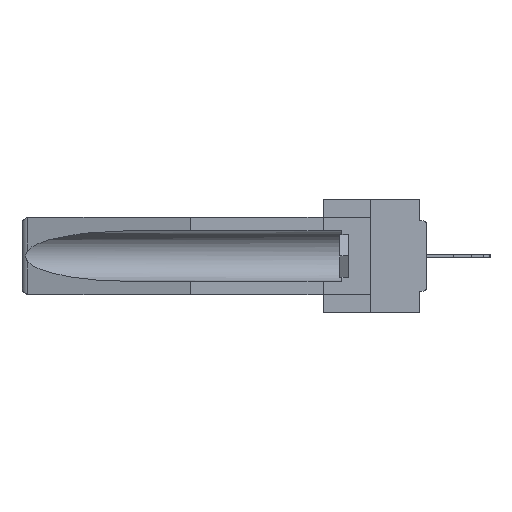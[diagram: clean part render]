
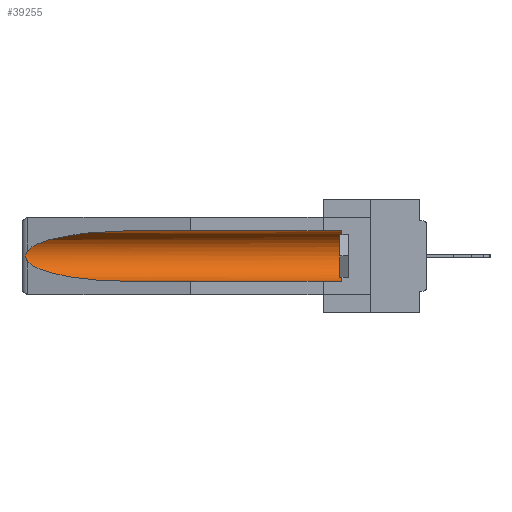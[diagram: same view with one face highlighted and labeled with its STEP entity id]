
A CAD part, left-side view. The second image highlights one B-rep face of the part: STEP entity #39255.
In plain terms, the highlighted cylindrical face has radius 2.857 mm (diameter 5.715 mm), a partial arc.
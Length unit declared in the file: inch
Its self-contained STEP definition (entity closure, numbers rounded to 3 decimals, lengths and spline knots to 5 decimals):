
#907 = CARTESIAN_POINT ( 'NONE',  ( 0.21114, 1.30732, -0.284 ) ) ;
#1145 = ORIENTED_EDGE ( 'NONE', *, *, #2730, .T. ) ;
#1500 = CARTESIAN_POINT ( 'NONE',  ( 0.155, 1.07973, -0.284 ) ) ;
#2730 = EDGE_CURVE ( 'NONE', #5577, #13444, #19659, .T. ) ;
#3007 = CARTESIAN_POINT ( 'NONE',  ( 0.26597, 1.5296, -0.19026 ) ) ;
#4577 = VERTEX_POINT ( 'NONE', #11105 ) ;
#5098 = VECTOR ( 'NONE', #37094, 39.37008 ) ;
#5509 = EDGE_CURVE ( 'NONE', #5577, #16531, #6895, .T. ) ;
#5577 = VERTEX_POINT ( 'NONE', #8643 ) ;
#5765 = CARTESIAN_POINT ( 'NONE',  ( 0.25451, 1.48313, -0.09465 ) ) ;
#6176 = CARTESIAN_POINT ( 'NONE',  ( 0.155, 1.07973, -0.059 ) ) ;
#6895 = LINE ( 'NONE', #29945, #38728 ) ;
#7158 = DIRECTION ( 'NONE',  ( 0., 1., 0. ) ) ;
#7533 = VERTEX_POINT ( 'NONE', #6176 ) ;
#7976 = ORIENTED_EDGE ( 'NONE', *, *, #5509, .F. ) ;
#8643 = CARTESIAN_POINT ( 'NONE',  ( 0.155, 0.126, -0.284 ) ) ;
#9172 = CARTESIAN_POINT ( 'NONE',  ( 0.26597, 1.52961, -0.15275 ) ) ;
#10484 = VERTEX_POINT ( 'NONE', #34458 ) ;
#11095 = DIRECTION ( 'NONE',  ( 0., -1., 0. ) ) ;
#11105 = CARTESIAN_POINT ( 'NONE',  ( 0.26537, 1.52718, -0.19328 ) ) ;
#11738 = B_SPLINE_CURVE_WITH_KNOTS ( 'NONE', 3,
 ( #18385, #9172, #33818, #15425, #36960, #18511, #40015, #21604, #3007, #24680 ),
 .UNSPECIFIED., .F., .F.,
 ( 4, 2, 2, 2, 4 ),
 ( 0., 0.00029, 0.00058, 0.00087, 0.00117 ),
 .UNSPECIFIED. ) ;
#13401 = LINE ( 'NONE', #21730, #5098 ) ;
#13444 = VERTEX_POINT ( 'NONE', #15749 ) ;
#13967 =( BOUNDED_CURVE ( )  B_SPLINE_CURVE ( 3, ( #38015, #19577, #907, #22663 ),
 .UNSPECIFIED., .F., .T. ) 
 B_SPLINE_CURVE_WITH_KNOTS ( ( 4, 4 ),
 ( 0.1948, 1.5708 ),
 .UNSPECIFIED. ) 
 CURVE ( )  GEOMETRIC_REPRESENTATION_ITEM ( )  RATIONAL_B_SPLINE_CURVE ( ( 1., 0.848, 0.848, 1. ) ) 
 REPRESENTATION_ITEM ( '' )  );
#14114 = AXIS2_PLACEMENT_3D ( 'NONE', #34916, #7158, #16513 ) ;
#14897 = ORIENTED_EDGE ( 'NONE', *, *, #30225, .T. ) ;
#15425 = CARTESIAN_POINT ( 'NONE',  ( 0.2673, 1.5327, -0.16383 ) ) ;
#15749 = CARTESIAN_POINT ( 'NONE',  ( 0.155, 0.126, -0.059 ) ) ;
#16513 = DIRECTION ( 'NONE',  ( 0., 0., 1. ) ) ;
#16531 = VERTEX_POINT ( 'NONE', #1500 ) ;
#16762 = EDGE_CURVE ( 'NONE', #7533, #10484, #32102, .T. ) ;
#16821 = EDGE_LOOP ( 'NONE', ( #34192, #40185, #24329, #7976, #1145, #14897 ) ) ;
#18385 = CARTESIAN_POINT ( 'NONE',  ( 0.26537, 1.52718, -0.14972 ) ) ;
#18511 = CARTESIAN_POINT ( 'NONE',  ( 0.2675, 1.53308, -0.17534 ) ) ;
#19577 = CARTESIAN_POINT ( 'NONE',  ( 0.25451, 1.48313, -0.24835 ) ) ;
#19659 = CIRCLE ( 'NONE', #37400, 0.1125 ) ;
#20816 = DIRECTION ( 'NONE',  ( 0., 1., 0. ) ) ;
#21604 = CARTESIAN_POINT ( 'NONE',  ( 0.26655, 1.53094, -0.18657 ) ) ;
#21730 = CARTESIAN_POINT ( 'NONE',  ( 0.155, -0.30754, -0.059 ) ) ;
#22663 = CARTESIAN_POINT ( 'NONE',  ( 0.155, 1.07973, -0.284 ) ) ;
#23661 = CYLINDRICAL_SURFACE ( 'NONE', #14114, 0.1125 ) ;
#24329 = ORIENTED_EDGE ( 'NONE', *, *, #34703, .T. ) ;
#24680 = CARTESIAN_POINT ( 'NONE',  ( 0.26537, 1.52718, -0.19328 ) ) ;
#27367 = CARTESIAN_POINT ( 'NONE',  ( 0.26537, 1.52718, -0.14972 ) ) ;
#28346 = EDGE_CURVE ( 'NONE', #10484, #4577, #11738, .T. ) ;
#29517 = CARTESIAN_POINT ( 'NONE',  ( 0.155, 0.126, -0.1715 ) ) ;
#29945 = CARTESIAN_POINT ( 'NONE',  ( 0.155, -0.30754, -0.284 ) ) ;
#30225 = EDGE_CURVE ( 'NONE', #13444, #7533, #13401, .T. ) ;
#30353 = CARTESIAN_POINT ( 'NONE',  ( 0.155, 1.07973, -0.059 ) ) ;
#32102 =( BOUNDED_CURVE ( )  B_SPLINE_CURVE ( 3, ( #30353, #33426, #5765, #27367 ),
 .UNSPECIFIED., .F., .F. ) 
 B_SPLINE_CURVE_WITH_KNOTS ( ( 4, 4 ),
 ( 4.71239, 6.08839 ),
 .UNSPECIFIED. ) 
 CURVE ( )  GEOMETRIC_REPRESENTATION_ITEM ( )  RATIONAL_B_SPLINE_CURVE ( ( 1., 0.848, 0.848, 1. ) ) 
 REPRESENTATION_ITEM ( '' )  );
#32607 = DIRECTION ( 'NONE',  ( 0., 0., 1. ) ) ;
#33426 = CARTESIAN_POINT ( 'NONE',  ( 0.21114, 1.30732, -0.059 ) ) ;
#33818 = CARTESIAN_POINT ( 'NONE',  ( 0.26654, 1.53092, -0.15636 ) ) ;
#34192 = ORIENTED_EDGE ( 'NONE', *, *, #16762, .T. ) ;
#34458 = CARTESIAN_POINT ( 'NONE',  ( 0.26537, 1.52718, -0.14972 ) ) ;
#34703 = EDGE_CURVE ( 'NONE', #4577, #16531, #13967, .T. ) ;
#34916 = CARTESIAN_POINT ( 'NONE',  ( 0.155, -0.30754, -0.1715 ) ) ;
#36960 = CARTESIAN_POINT ( 'NONE',  ( 0.2675, 1.53308, -0.16763 ) ) ;
#37094 = DIRECTION ( 'NONE',  ( 0., 1., 0. ) ) ;
#37400 = AXIS2_PLACEMENT_3D ( 'NONE', #29517, #11095, #32607 ) ;
#38015 = CARTESIAN_POINT ( 'NONE',  ( 0.26537, 1.52718, -0.19328 ) ) ;
#38728 = VECTOR ( 'NONE', #20816, 39.37008 ) ;
#39255 = ADVANCED_FACE ( 'NONE', ( #40034 ), #23661, .F. ) ;
#40015 = CARTESIAN_POINT ( 'NONE',  ( 0.2673, 1.53269, -0.17917 ) ) ;
#40034 = FACE_OUTER_BOUND ( 'NONE', #16821, .T. ) ;
#40185 = ORIENTED_EDGE ( 'NONE', *, *, #28346, .T. ) ;
